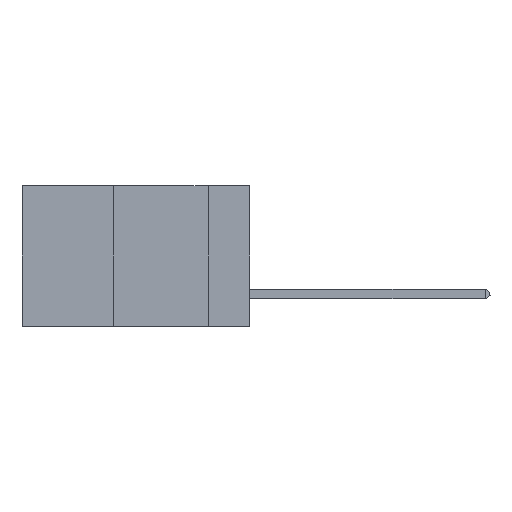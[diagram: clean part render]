
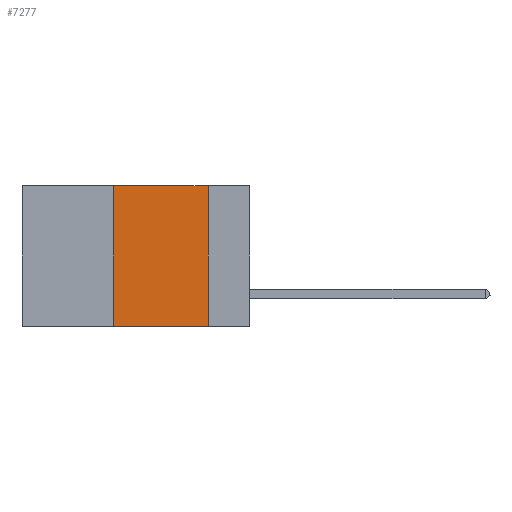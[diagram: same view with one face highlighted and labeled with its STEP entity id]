
A CAD part, left-side view. The second image highlights one B-rep face of the part: STEP entity #7277.
In plain terms, the highlighted planar face has unit normal (-1, 0, 0).
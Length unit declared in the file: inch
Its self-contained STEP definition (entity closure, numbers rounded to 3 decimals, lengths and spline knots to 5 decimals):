
#1252 = AXIS2_PLACEMENT_3D ( 'NONE', #6867, #5642, #5378 ) ;
#1934 = CARTESIAN_POINT ( 'NONE',  ( 0., 0.36, 0. ) ) ;
#2043 = LINE ( 'NONE', #4622, #15679 ) ;
#2500 = ORIENTED_EDGE ( 'NONE', *, *, #13315, .F. ) ;
#3590 = FACE_OUTER_BOUND ( 'NONE', #15888, .T. ) ;
#3759 = VERTEX_POINT ( 'NONE', #9051 ) ;
#4242 = ORIENTED_EDGE ( 'NONE', *, *, #20763, .F. ) ;
#4264 = LINE ( 'NONE', #1934, #14143 ) ;
#4622 = CARTESIAN_POINT ( 'NONE',  ( 0., 0.6, 0. ) ) ;
#5378 = DIRECTION ( 'NONE',  ( 0., 0., -1. ) ) ;
#5642 = DIRECTION ( 'NONE',  ( 1., 0., 0. ) ) ;
#6867 = CARTESIAN_POINT ( 'NONE',  ( 0., 0.6, 0. ) ) ;
#6945 = PLANE ( 'NONE',  #1252 ) ;
#7225 = EDGE_CURVE ( 'NONE', #3759, #15146, #2043, .T. ) ;
#7277 = ADVANCED_FACE ( 'NONE', ( #3590 ), #6945, .F. ) ;
#8645 = DIRECTION ( 'NONE',  ( 0., -1., 0. ) ) ;
#8861 = DIRECTION ( 'NONE',  ( 0., 0., -1. ) ) ;
#9051 = CARTESIAN_POINT ( 'NONE',  ( 0., 0.36, 0. ) ) ;
#9516 = VECTOR ( 'NONE', #8645, 39.37008 ) ;
#9821 = CARTESIAN_POINT ( 'NONE',  ( 0., 0.11, -0.37 ) ) ;
#10549 = LINE ( 'NONE', #15319, #17924 ) ;
#11484 = CARTESIAN_POINT ( 'NONE',  ( 0., 0.11, 0. ) ) ;
#13315 = EDGE_CURVE ( 'NONE', #15146, #24478, #10549, .T. ) ;
#13772 = ORIENTED_EDGE ( 'NONE', *, *, #7225, .F. ) ;
#13959 = DIRECTION ( 'NONE',  ( 0., 0., 1. ) ) ;
#14143 = VECTOR ( 'NONE', #13959, 39.37008 ) ;
#14374 = DIRECTION ( 'NONE',  ( 0., -1., 0. ) ) ;
#15146 = VERTEX_POINT ( 'NONE', #11484 ) ;
#15319 = CARTESIAN_POINT ( 'NONE',  ( 0., 0.11, 0. ) ) ;
#15679 = VECTOR ( 'NONE', #14374, 39.37008 ) ;
#15888 = EDGE_LOOP ( 'NONE', ( #2500, #13772, #4242, #20429 ) ) ;
#16348 = CARTESIAN_POINT ( 'NONE',  ( 0., 0.36, -0.37 ) ) ;
#17924 = VECTOR ( 'NONE', #8861, 39.37008 ) ;
#20420 = CARTESIAN_POINT ( 'NONE',  ( 0., 0.6, -0.37 ) ) ;
#20429 = ORIENTED_EDGE ( 'NONE', *, *, #25542, .T. ) ;
#20763 = EDGE_CURVE ( 'NONE', #24925, #3759, #4264, .T. ) ;
#24478 = VERTEX_POINT ( 'NONE', #9821 ) ;
#24925 = VERTEX_POINT ( 'NONE', #16348 ) ;
#25261 = LINE ( 'NONE', #20420, #9516 ) ;
#25542 = EDGE_CURVE ( 'NONE', #24925, #24478, #25261, .T. ) ;
